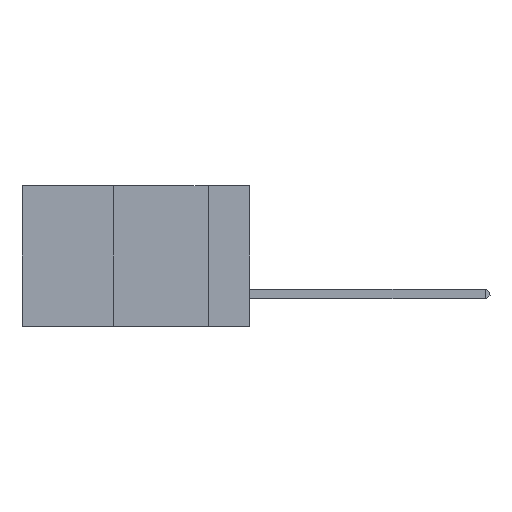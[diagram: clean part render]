
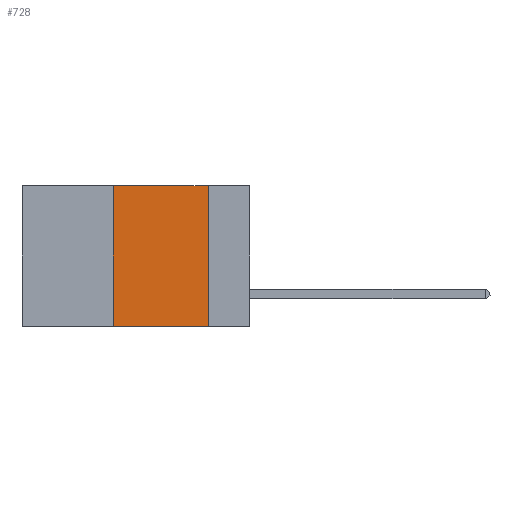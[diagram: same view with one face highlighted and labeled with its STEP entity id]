
A CAD part, left-side view. The second image highlights one B-rep face of the part: STEP entity #728.
In plain terms, the highlighted planar face has unit normal (-1, 0, 0).
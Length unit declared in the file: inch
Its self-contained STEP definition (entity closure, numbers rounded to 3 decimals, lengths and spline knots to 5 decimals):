
#728 = ADVANCED_FACE ( 'NONE', ( #3957 ), #11464, .F. ) ;
#914 = DIRECTION ( 'NONE',  ( 0., -1., 0. ) ) ;
#1073 = VERTEX_POINT ( 'NONE', #2495 ) ;
#1225 = DIRECTION ( 'NONE',  ( 1., 0., 0. ) ) ;
#2075 = ORIENTED_EDGE ( 'NONE', *, *, #6508, .F. ) ;
#2358 = ORIENTED_EDGE ( 'NONE', *, *, #7548, .F. ) ;
#2495 = CARTESIAN_POINT ( 'NONE',  ( 0., 0.11, -0.37 ) ) ;
#2670 = VECTOR ( 'NONE', #6435, 39.37008 ) ;
#3295 = DIRECTION ( 'NONE',  ( 0., 0., -1. ) ) ;
#3957 = FACE_OUTER_BOUND ( 'NONE', #6658, .T. ) ;
#4156 = LINE ( 'NONE', #5377, #11038 ) ;
#4157 = CARTESIAN_POINT ( 'NONE',  ( 0., 0.36, 0. ) ) ;
#4655 = DIRECTION ( 'NONE',  ( 0., -1., 0. ) ) ;
#5377 = CARTESIAN_POINT ( 'NONE',  ( 0., 0.11, 0. ) ) ;
#5814 = EDGE_CURVE ( 'NONE', #9319, #1073, #11845, .T. ) ;
#6205 = LINE ( 'NONE', #10698, #8136 ) ;
#6435 = DIRECTION ( 'NONE',  ( 0., 0., 1. ) ) ;
#6508 = EDGE_CURVE ( 'NONE', #9319, #9779, #11983, .T. ) ;
#6658 = EDGE_LOOP ( 'NONE', ( #2358, #9880, #2075, #12044 ) ) ;
#7548 = EDGE_CURVE ( 'NONE', #11785, #1073, #4156, .T. ) ;
#7637 = CARTESIAN_POINT ( 'NONE',  ( 0., 0.36, -0.37 ) ) ;
#8136 = VECTOR ( 'NONE', #4655, 39.37008 ) ;
#8246 = CARTESIAN_POINT ( 'NONE',  ( 0., 0.6, -0.37 ) ) ;
#8779 = EDGE_CURVE ( 'NONE', #9779, #11785, #6205, .T. ) ;
#9166 = VECTOR ( 'NONE', #914, 39.37008 ) ;
#9319 = VERTEX_POINT ( 'NONE', #7637 ) ;
#9354 = CARTESIAN_POINT ( 'NONE',  ( 0., 0.36, 0. ) ) ;
#9779 = VERTEX_POINT ( 'NONE', #4157 ) ;
#9880 = ORIENTED_EDGE ( 'NONE', *, *, #8779, .F. ) ;
#10367 = DIRECTION ( 'NONE',  ( 0., 0., -1. ) ) ;
#10698 = CARTESIAN_POINT ( 'NONE',  ( 0., 0.6, 0. ) ) ;
#10950 = CARTESIAN_POINT ( 'NONE',  ( 0., 0.11, 0. ) ) ;
#11038 = VECTOR ( 'NONE', #3295, 39.37008 ) ;
#11282 = CARTESIAN_POINT ( 'NONE',  ( 0., 0.6, 0. ) ) ;
#11464 = PLANE ( 'NONE',  #13179 ) ;
#11785 = VERTEX_POINT ( 'NONE', #10950 ) ;
#11845 = LINE ( 'NONE', #8246, #9166 ) ;
#11983 = LINE ( 'NONE', #9354, #2670 ) ;
#12044 = ORIENTED_EDGE ( 'NONE', *, *, #5814, .T. ) ;
#13179 = AXIS2_PLACEMENT_3D ( 'NONE', #11282, #1225, #10367 ) ;
